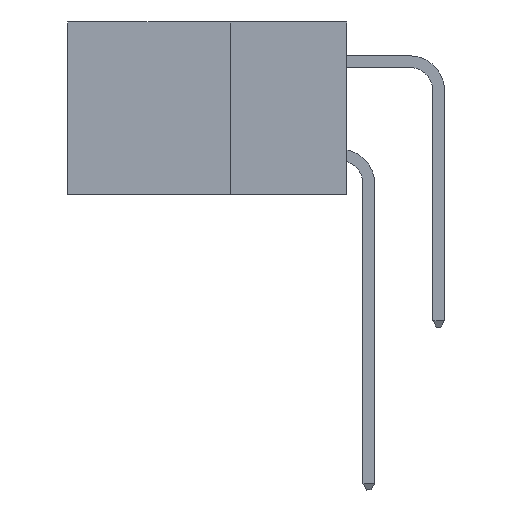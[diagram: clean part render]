
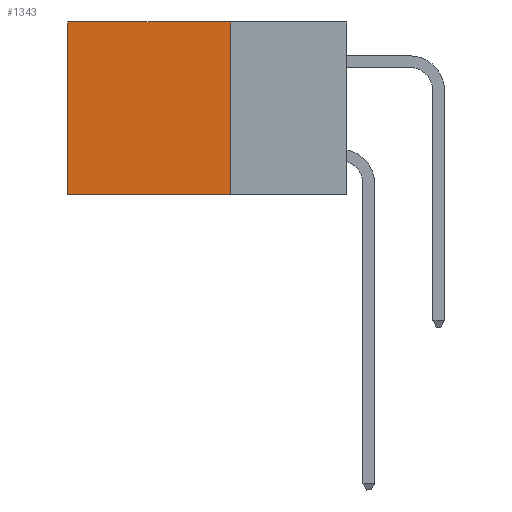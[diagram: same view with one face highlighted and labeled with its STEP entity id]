
A CAD part, left-side view. The second image highlights one B-rep face of the part: STEP entity #1343.
In plain terms, the highlighted planar face has unit normal (-1, 0, 0).
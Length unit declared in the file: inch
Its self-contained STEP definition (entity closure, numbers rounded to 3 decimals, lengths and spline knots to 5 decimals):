
#566 = ORIENTED_EDGE ( 'NONE', *, *, #2828, .F. ) ;
#1343 = ADVANCED_FACE ( 'NONE', ( #7724 ), #13226, .F. ) ;
#1741 = VECTOR ( 'NONE', #2925, 39.37008 ) ;
#2828 = EDGE_CURVE ( 'NONE', #9260, #4352, #14971, .T. ) ;
#2925 = DIRECTION ( 'NONE',  ( 0., 0., -1. ) ) ;
#3809 = CARTESIAN_POINT ( 'NONE',  ( 0.2875, 0.25, -0.37 ) ) ;
#4322 = LINE ( 'NONE', #4371, #10505 ) ;
#4336 = EDGE_CURVE ( 'NONE', #11068, #5881, #11717, .T. ) ;
#4352 = VERTEX_POINT ( 'NONE', #3809 ) ;
#4371 = CARTESIAN_POINT ( 'NONE',  ( 0.2875, 0.25, -0.37 ) ) ;
#4429 = CARTESIAN_POINT ( 'NONE',  ( 0.2875, 0.25, 0. ) ) ;
#4466 = CARTESIAN_POINT ( 'NONE',  ( 0.2875, 0.6, -0.37 ) ) ;
#4624 = DIRECTION ( 'NONE',  ( 0., 1., 0. ) ) ;
#5138 = EDGE_CURVE ( 'NONE', #9260, #11068, #17684, .T. ) ;
#5514 = VECTOR ( 'NONE', #7343, 39.37008 ) ;
#5881 = VERTEX_POINT ( 'NONE', #4466 ) ;
#6661 = CARTESIAN_POINT ( 'NONE',  ( 0.2875, 0.25, 0. ) ) ;
#6717 = ORIENTED_EDGE ( 'NONE', *, *, #4336, .T. ) ;
#6975 = ORIENTED_EDGE ( 'NONE', *, *, #16474, .F. ) ;
#7343 = DIRECTION ( 'NONE',  ( 0., 0., -1. ) ) ;
#7456 = DIRECTION ( 'NONE',  ( 1., 0., 0. ) ) ;
#7724 = FACE_OUTER_BOUND ( 'NONE', #8474, .T. ) ;
#8474 = EDGE_LOOP ( 'NONE', ( #6717, #6975, #566, #17364 ) ) ;
#9260 = VERTEX_POINT ( 'NONE', #4429 ) ;
#10505 = VECTOR ( 'NONE', #4624, 39.37008 ) ;
#11068 = VERTEX_POINT ( 'NONE', #15004 ) ;
#11717 = LINE ( 'NONE', #14946, #1741 ) ;
#13167 = DIRECTION ( 'NONE',  ( 0., 0., -1. ) ) ;
#13226 = PLANE ( 'NONE',  #15789 ) ;
#14434 = CARTESIAN_POINT ( 'NONE',  ( 0.2875, 0.25, 0. ) ) ;
#14946 = CARTESIAN_POINT ( 'NONE',  ( 0.2875, 0.6, 0. ) ) ;
#14971 = LINE ( 'NONE', #14434, #5514 ) ;
#15004 = CARTESIAN_POINT ( 'NONE',  ( 0.2875, 0.6, 0. ) ) ;
#15789 = AXIS2_PLACEMENT_3D ( 'NONE', #16097, #7456, #13167 ) ;
#16097 = CARTESIAN_POINT ( 'NONE',  ( 0.2875, 0.25, 0. ) ) ;
#16474 = EDGE_CURVE ( 'NONE', #4352, #5881, #4322, .T. ) ;
#17364 = ORIENTED_EDGE ( 'NONE', *, *, #5138, .T. ) ;
#17684 = LINE ( 'NONE', #6661, #17907 ) ;
#17870 = DIRECTION ( 'NONE',  ( 0., 1., 0. ) ) ;
#17907 = VECTOR ( 'NONE', #17870, 39.37008 ) ;
